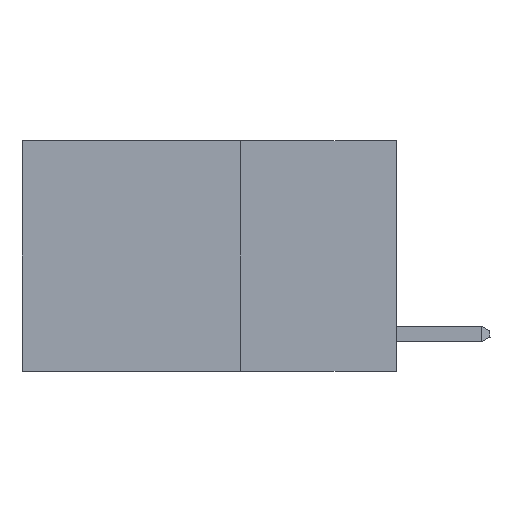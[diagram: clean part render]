
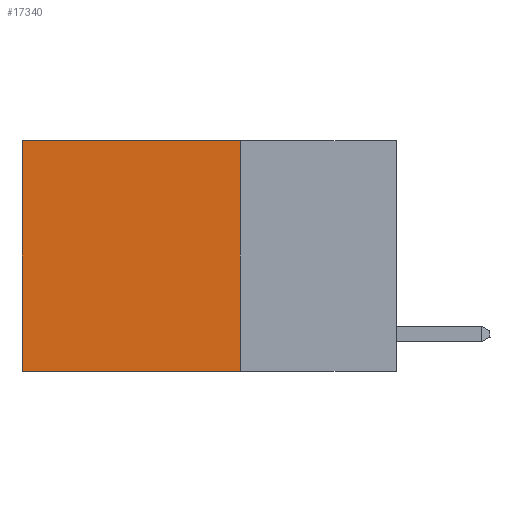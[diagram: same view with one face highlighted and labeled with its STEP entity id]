
A CAD part, left-side view. The second image highlights one B-rep face of the part: STEP entity #17340.
In plain terms, the highlighted planar face has unit normal (-1, 0, 0).
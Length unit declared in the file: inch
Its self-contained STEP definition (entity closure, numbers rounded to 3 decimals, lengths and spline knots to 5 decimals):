
#604 = VECTOR ( 'NONE', #27276, 39.37008 ) ;
#826 = DIRECTION ( 'NONE',  ( 0., 0., -1. ) ) ;
#2063 = CARTESIAN_POINT ( 'NONE',  ( 0.2625, 0.25, -0.37 ) ) ;
#3390 = AXIS2_PLACEMENT_3D ( 'NONE', #9876, #25994, #12243 ) ;
#4198 = EDGE_CURVE ( 'NONE', #6627, #15351, #21990, .T. ) ;
#4352 = DIRECTION ( 'NONE',  ( 0., 0., -1. ) ) ;
#4531 = EDGE_CURVE ( 'NONE', #26862, #27912, #25562, .T. ) ;
#6549 = CARTESIAN_POINT ( 'NONE',  ( 0.2625, 0.25, 0. ) ) ;
#6627 = VERTEX_POINT ( 'NONE', #14258 ) ;
#6691 = CARTESIAN_POINT ( 'NONE',  ( 0.2625, 0.25, -0.37 ) ) ;
#8921 = CARTESIAN_POINT ( 'NONE',  ( 0.2625, 0.25, 0. ) ) ;
#9033 = DIRECTION ( 'NONE',  ( 0., 1., 0. ) ) ;
#9876 = CARTESIAN_POINT ( 'NONE',  ( 0.2625, 0.25, 0. ) ) ;
#10821 = ORIENTED_EDGE ( 'NONE', *, *, #29406, .T. ) ;
#11009 = ORIENTED_EDGE ( 'NONE', *, *, #4531, .F. ) ;
#11093 = ORIENTED_EDGE ( 'NONE', *, *, #4198, .T. ) ;
#11356 = EDGE_LOOP ( 'NONE', ( #11093, #18502, #11009, #10821 ) ) ;
#12152 = CARTESIAN_POINT ( 'NONE',  ( 0.2625, 0.25, 0. ) ) ;
#12243 = DIRECTION ( 'NONE',  ( 0., 0., -1. ) ) ;
#12507 = CARTESIAN_POINT ( 'NONE',  ( 0.2625, 0.6, 0. ) ) ;
#14258 = CARTESIAN_POINT ( 'NONE',  ( 0.2625, 0.6, 0. ) ) ;
#14975 = LINE ( 'NONE', #6691, #26446 ) ;
#15177 = VECTOR ( 'NONE', #826, 39.37008 ) ;
#15351 = VERTEX_POINT ( 'NONE', #17889 ) ;
#16762 = PLANE ( 'NONE',  #3390 ) ;
#17340 = ADVANCED_FACE ( 'NONE', ( #28128 ), #16762, .F. ) ;
#17889 = CARTESIAN_POINT ( 'NONE',  ( 0.2625, 0.6, -0.37 ) ) ;
#18502 = ORIENTED_EDGE ( 'NONE', *, *, #27887, .F. ) ;
#21990 = LINE ( 'NONE', #12507, #15177 ) ;
#24827 = VECTOR ( 'NONE', #4352, 39.37008 ) ;
#25562 = LINE ( 'NONE', #8921, #24827 ) ;
#25994 = DIRECTION ( 'NONE',  ( 1., 0., 0. ) ) ;
#25999 = LINE ( 'NONE', #6549, #604 ) ;
#26446 = VECTOR ( 'NONE', #9033, 39.37008 ) ;
#26862 = VERTEX_POINT ( 'NONE', #12152 ) ;
#27276 = DIRECTION ( 'NONE',  ( 0., 1., 0. ) ) ;
#27887 = EDGE_CURVE ( 'NONE', #27912, #15351, #14975, .T. ) ;
#27912 = VERTEX_POINT ( 'NONE', #2063 ) ;
#28128 = FACE_OUTER_BOUND ( 'NONE', #11356, .T. ) ;
#29406 = EDGE_CURVE ( 'NONE', #26862, #6627, #25999, .T. ) ;
